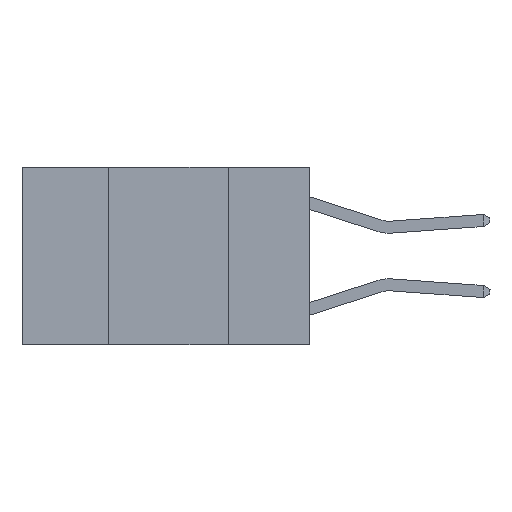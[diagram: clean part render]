
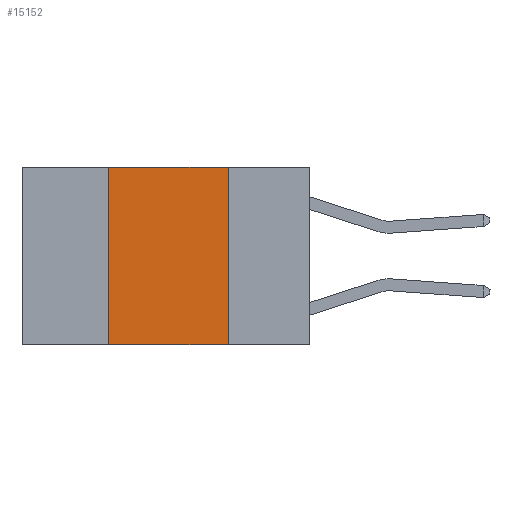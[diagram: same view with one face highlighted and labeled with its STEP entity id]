
A CAD part, left-side view. The second image highlights one B-rep face of the part: STEP entity #15152.
In plain terms, the highlighted planar face has unit normal (-1, 0, 0).
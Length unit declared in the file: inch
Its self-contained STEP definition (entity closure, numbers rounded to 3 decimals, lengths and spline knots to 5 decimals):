
#781 = ORIENTED_EDGE ( 'NONE', *, *, #18347, .F. ) ;
#2270 = CARTESIAN_POINT ( 'NONE',  ( 0., 0.42, 0. ) ) ;
#2497 = CARTESIAN_POINT ( 'NONE',  ( 0., 0.17, -0.37 ) ) ;
#3030 = CARTESIAN_POINT ( 'NONE',  ( 0., 0.17, 0. ) ) ;
#3101 = VECTOR ( 'NONE', #28420, 39.37008 ) ;
#4846 = ORIENTED_EDGE ( 'NONE', *, *, #14874, .F. ) ;
#7120 = EDGE_CURVE ( 'NONE', #12044, #24847, #18906, .T. ) ;
#8051 = DIRECTION ( 'NONE',  ( 0., -1., 0. ) ) ;
#8274 = LINE ( 'NONE', #13406, #17497 ) ;
#8911 = EDGE_LOOP ( 'NONE', ( #781, #4846, #27372, #18569 ) ) ;
#10584 = CARTESIAN_POINT ( 'NONE',  ( 0., 0.6, 0. ) ) ;
#12044 = VERTEX_POINT ( 'NONE', #13842 ) ;
#13406 = CARTESIAN_POINT ( 'NONE',  ( 0., 0.17, 0. ) ) ;
#13842 = CARTESIAN_POINT ( 'NONE',  ( 0., 0.42, -0.37 ) ) ;
#13954 = CARTESIAN_POINT ( 'NONE',  ( 0., 0.6, -0.37 ) ) ;
#14874 = EDGE_CURVE ( 'NONE', #24847, #30765, #23473, .T. ) ;
#15152 = ADVANCED_FACE ( 'NONE', ( #30349 ), #15421, .F. ) ;
#15421 = PLANE ( 'NONE',  #17995 ) ;
#15459 = CARTESIAN_POINT ( 'NONE',  ( 0., 0.6, 0. ) ) ;
#15738 = DIRECTION ( 'NONE',  ( 0., 0., -1. ) ) ;
#16713 = EDGE_CURVE ( 'NONE', #12044, #31152, #24244, .T. ) ;
#17497 = VECTOR ( 'NONE', #28516, 39.37008 ) ;
#17995 = AXIS2_PLACEMENT_3D ( 'NONE', #10584, #25222, #15738 ) ;
#18347 = EDGE_CURVE ( 'NONE', #30765, #31152, #8274, .T. ) ;
#18569 = ORIENTED_EDGE ( 'NONE', *, *, #16713, .T. ) ;
#18906 = LINE ( 'NONE', #23722, #28717 ) ;
#23473 = LINE ( 'NONE', #15459, #25500 ) ;
#23722 = CARTESIAN_POINT ( 'NONE',  ( 0., 0.42, 0. ) ) ;
#24244 = LINE ( 'NONE', #13954, #3101 ) ;
#24847 = VERTEX_POINT ( 'NONE', #2270 ) ;
#25222 = DIRECTION ( 'NONE',  ( 1., 0., 0. ) ) ;
#25500 = VECTOR ( 'NONE', #8051, 39.37008 ) ;
#27372 = ORIENTED_EDGE ( 'NONE', *, *, #7120, .F. ) ;
#28420 = DIRECTION ( 'NONE',  ( 0., -1., 0. ) ) ;
#28516 = DIRECTION ( 'NONE',  ( 0., 0., -1. ) ) ;
#28717 = VECTOR ( 'NONE', #31253, 39.37008 ) ;
#30349 = FACE_OUTER_BOUND ( 'NONE', #8911, .T. ) ;
#30765 = VERTEX_POINT ( 'NONE', #3030 ) ;
#31152 = VERTEX_POINT ( 'NONE', #2497 ) ;
#31253 = DIRECTION ( 'NONE',  ( 0., 0., 1. ) ) ;
